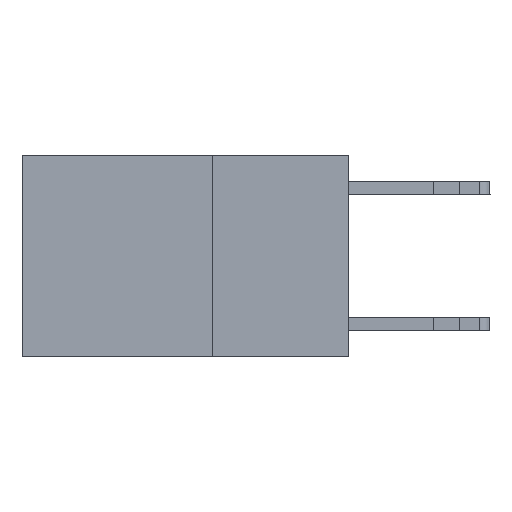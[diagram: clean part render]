
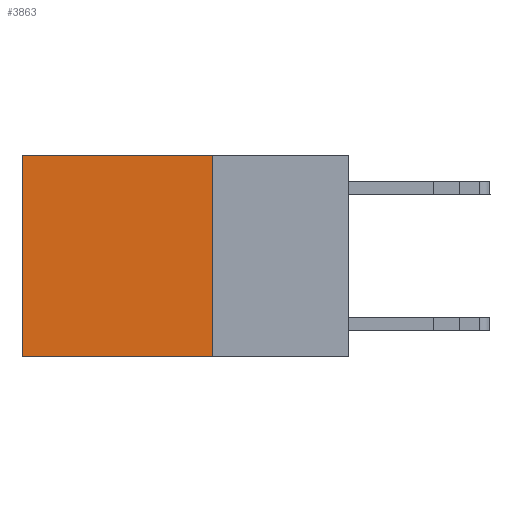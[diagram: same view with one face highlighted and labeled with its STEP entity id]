
A CAD part, left-side view. The second image highlights one B-rep face of the part: STEP entity #3863.
In plain terms, the highlighted planar face has unit normal (-1, 0, 0).
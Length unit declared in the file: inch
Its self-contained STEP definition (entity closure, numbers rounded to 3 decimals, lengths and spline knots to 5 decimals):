
#762 = EDGE_CURVE ( 'NONE', #14180, #6026, #5620, .T. ) ;
#1214 = CARTESIAN_POINT ( 'NONE',  ( 0.2625, 0.6, -0.37 ) ) ;
#1727 = VECTOR ( 'NONE', #1898, 39.37008 ) ;
#1898 = DIRECTION ( 'NONE',  ( 0., 0., -1. ) ) ;
#3083 = CARTESIAN_POINT ( 'NONE',  ( 0.2625, 0.25, 0. ) ) ;
#3760 = CARTESIAN_POINT ( 'NONE',  ( 0.2625, 0.6, 0. ) ) ;
#3863 = ADVANCED_FACE ( 'NONE', ( #14355 ), #12725, .F. ) ;
#3958 = ORIENTED_EDGE ( 'NONE', *, *, #8454, .T. ) ;
#4244 = CARTESIAN_POINT ( 'NONE',  ( 0.2625, 0.25, -0.37 ) ) ;
#4741 = CARTESIAN_POINT ( 'NONE',  ( 0.2625, 0.25, 0. ) ) ;
#4825 = VERTEX_POINT ( 'NONE', #17450 ) ;
#5335 = VECTOR ( 'NONE', #9324, 39.37008 ) ;
#5620 = LINE ( 'NONE', #11150, #15218 ) ;
#6026 = VERTEX_POINT ( 'NONE', #8602 ) ;
#6417 = ORIENTED_EDGE ( 'NONE', *, *, #14400, .F. ) ;
#8454 = EDGE_CURVE ( 'NONE', #6026, #9779, #16207, .T. ) ;
#8602 = CARTESIAN_POINT ( 'NONE',  ( 0.2625, 0.6, 0. ) ) ;
#9324 = DIRECTION ( 'NONE',  ( 0., 0., -1. ) ) ;
#9779 = VERTEX_POINT ( 'NONE', #1214 ) ;
#10184 = DIRECTION ( 'NONE',  ( 1., 0., 0. ) ) ;
#10540 = CARTESIAN_POINT ( 'NONE',  ( 0.2625, 0.25, 0. ) ) ;
#11150 = CARTESIAN_POINT ( 'NONE',  ( 0.2625, 0.25, 0. ) ) ;
#11301 = DIRECTION ( 'NONE',  ( 0., 1., 0. ) ) ;
#11429 = LINE ( 'NONE', #3083, #1727 ) ;
#11966 = AXIS2_PLACEMENT_3D ( 'NONE', #4741, #10184, #15809 ) ;
#12725 = PLANE ( 'NONE',  #11966 ) ;
#13782 = LINE ( 'NONE', #4244, #16542 ) ;
#14098 = ORIENTED_EDGE ( 'NONE', *, *, #14580, .F. ) ;
#14180 = VERTEX_POINT ( 'NONE', #10540 ) ;
#14355 = FACE_OUTER_BOUND ( 'NONE', #17886, .T. ) ;
#14400 = EDGE_CURVE ( 'NONE', #14180, #4825, #11429, .T. ) ;
#14580 = EDGE_CURVE ( 'NONE', #4825, #9779, #13782, .T. ) ;
#15218 = VECTOR ( 'NONE', #16696, 39.37008 ) ;
#15809 = DIRECTION ( 'NONE',  ( 0., 0., -1. ) ) ;
#16207 = LINE ( 'NONE', #3760, #5335 ) ;
#16542 = VECTOR ( 'NONE', #11301, 39.37008 ) ;
#16696 = DIRECTION ( 'NONE',  ( 0., 1., 0. ) ) ;
#17431 = ORIENTED_EDGE ( 'NONE', *, *, #762, .T. ) ;
#17450 = CARTESIAN_POINT ( 'NONE',  ( 0.2625, 0.25, -0.37 ) ) ;
#17886 = EDGE_LOOP ( 'NONE', ( #3958, #14098, #6417, #17431 ) ) ;
